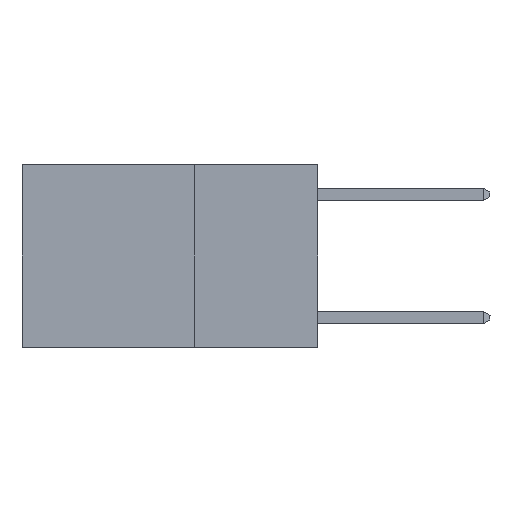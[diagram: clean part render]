
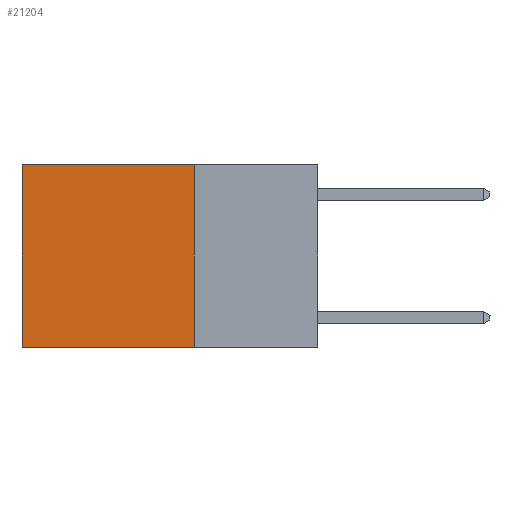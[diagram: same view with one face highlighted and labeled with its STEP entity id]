
A CAD part, left-side view. The second image highlights one B-rep face of the part: STEP entity #21204.
In plain terms, the highlighted planar face has unit normal (-1, 0, 0).
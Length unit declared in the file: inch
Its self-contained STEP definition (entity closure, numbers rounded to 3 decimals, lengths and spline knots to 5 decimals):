
#855 = DIRECTION ( 'NONE',  ( 0., 1., 0. ) ) ;
#1691 = ORIENTED_EDGE ( 'NONE', *, *, #28642, .F. ) ;
#1754 = EDGE_CURVE ( 'NONE', #16593, #25544, #28490, .T. ) ;
#3442 = EDGE_LOOP ( 'NONE', ( #8821, #11572, #1691, #7130 ) ) ;
#6597 = CARTESIAN_POINT ( 'NONE',  ( 0.2625, 0.6, 0. ) ) ;
#7130 = ORIENTED_EDGE ( 'NONE', *, *, #20067, .T. ) ;
#7572 = PLANE ( 'NONE',  #25681 ) ;
#8096 = EDGE_CURVE ( 'NONE', #13281, #25544, #24772, .T. ) ;
#8593 = DIRECTION ( 'NONE',  ( 0., 1., 0. ) ) ;
#8821 = ORIENTED_EDGE ( 'NONE', *, *, #1754, .T. ) ;
#9401 = VERTEX_POINT ( 'NONE', #11822 ) ;
#9624 = CARTESIAN_POINT ( 'NONE',  ( 0.2625, 0.25, 0. ) ) ;
#9768 = DIRECTION ( 'NONE',  ( 1., 0., 0. ) ) ;
#10101 = CARTESIAN_POINT ( 'NONE',  ( 0.2625, 0.25, 0. ) ) ;
#10719 = CARTESIAN_POINT ( 'NONE',  ( 0.2625, 0.25, -0.37 ) ) ;
#11572 = ORIENTED_EDGE ( 'NONE', *, *, #8096, .F. ) ;
#11822 = CARTESIAN_POINT ( 'NONE',  ( 0.2625, 0.25, 0. ) ) ;
#12060 = DIRECTION ( 'NONE',  ( 0., 0., -1. ) ) ;
#12611 = VECTOR ( 'NONE', #855, 39.37008 ) ;
#13281 = VERTEX_POINT ( 'NONE', #24985 ) ;
#13995 = FACE_OUTER_BOUND ( 'NONE', #3442, .T. ) ;
#16593 = VERTEX_POINT ( 'NONE', #6597 ) ;
#19017 = DIRECTION ( 'NONE',  ( 0., 0., -1. ) ) ;
#19795 = CARTESIAN_POINT ( 'NONE',  ( 0.2625, 0.6, -0.37 ) ) ;
#20067 = EDGE_CURVE ( 'NONE', #9401, #16593, #26595, .T. ) ;
#21180 = VECTOR ( 'NONE', #8593, 39.37008 ) ;
#21204 = ADVANCED_FACE ( 'NONE', ( #13995 ), #7572, .F. ) ;
#22414 = VECTOR ( 'NONE', #19017, 39.37008 ) ;
#23374 = VECTOR ( 'NONE', #28142, 39.37008 ) ;
#23453 = CARTESIAN_POINT ( 'NONE',  ( 0.2625, 0.25, 0. ) ) ;
#24772 = LINE ( 'NONE', #10719, #21180 ) ;
#24985 = CARTESIAN_POINT ( 'NONE',  ( 0.2625, 0.25, -0.37 ) ) ;
#25544 = VERTEX_POINT ( 'NONE', #19795 ) ;
#25681 = AXIS2_PLACEMENT_3D ( 'NONE', #23453, #9768, #12060 ) ;
#26595 = LINE ( 'NONE', #10101, #12611 ) ;
#28015 = CARTESIAN_POINT ( 'NONE',  ( 0.2625, 0.6, 0. ) ) ;
#28142 = DIRECTION ( 'NONE',  ( 0., 0., -1. ) ) ;
#28490 = LINE ( 'NONE', #28015, #22414 ) ;
#28642 = EDGE_CURVE ( 'NONE', #9401, #13281, #29472, .T. ) ;
#29472 = LINE ( 'NONE', #9624, #23374 ) ;
